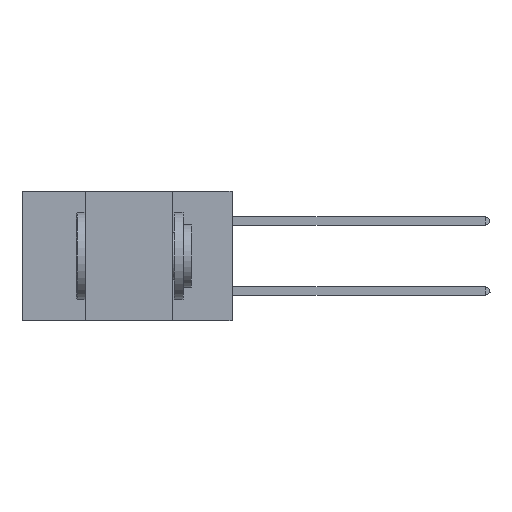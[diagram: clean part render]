
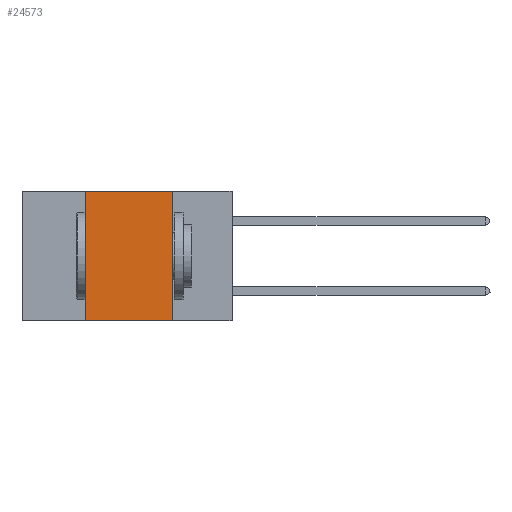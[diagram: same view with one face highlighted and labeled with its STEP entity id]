
A CAD part, left-side view. The second image highlights one B-rep face of the part: STEP entity #24573.
In plain terms, the highlighted planar face has unit normal (-1, 0, 0).
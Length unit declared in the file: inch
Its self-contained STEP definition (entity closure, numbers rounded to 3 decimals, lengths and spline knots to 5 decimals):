
#887 = CARTESIAN_POINT ( 'NONE',  ( 0., 0.42, -0.37 ) ) ;
#1390 = FACE_OUTER_BOUND ( 'NONE', #9276, .T. ) ;
#1487 = ORIENTED_EDGE ( 'NONE', *, *, #33273, .F. ) ;
#3387 = CARTESIAN_POINT ( 'NONE',  ( 0., 0.6, -0.37 ) ) ;
#4075 = VERTEX_POINT ( 'NONE', #34671 ) ;
#4514 = DIRECTION ( 'NONE',  ( 0., -1., 0. ) ) ;
#5145 = LINE ( 'NONE', #28663, #33664 ) ;
#7733 = DIRECTION ( 'NONE',  ( 0., 0., -1. ) ) ;
#7948 = VERTEX_POINT ( 'NONE', #12172 ) ;
#8188 = LINE ( 'NONE', #35156, #29239 ) ;
#9276 = EDGE_LOOP ( 'NONE', ( #1487, #20890, #13299, #32696 ) ) ;
#9795 = DIRECTION ( 'NONE',  ( 0., 0., 1. ) ) ;
#12172 = CARTESIAN_POINT ( 'NONE',  ( 0., 0.17, -0.37 ) ) ;
#13299 = ORIENTED_EDGE ( 'NONE', *, *, #27723, .F. ) ;
#16791 = DIRECTION ( 'NONE',  ( 0., 0., -1. ) ) ;
#17691 = VERTEX_POINT ( 'NONE', #887 ) ;
#17875 = LINE ( 'NONE', #3387, #32111 ) ;
#17896 = CARTESIAN_POINT ( 'NONE',  ( 0., 0.6, 0. ) ) ;
#18931 = EDGE_CURVE ( 'NONE', #4075, #21295, #27605, .T. ) ;
#20890 = ORIENTED_EDGE ( 'NONE', *, *, #18931, .F. ) ;
#21270 = AXIS2_PLACEMENT_3D ( 'NONE', #24106, #21484, #7733 ) ;
#21295 = VERTEX_POINT ( 'NONE', #23881 ) ;
#21484 = DIRECTION ( 'NONE',  ( 1., 0., 0. ) ) ;
#22049 = VECTOR ( 'NONE', #4514, 39.37008 ) ;
#22557 = EDGE_CURVE ( 'NONE', #17691, #7948, #17875, .T. ) ;
#23881 = CARTESIAN_POINT ( 'NONE',  ( 0., 0.17, 0. ) ) ;
#24106 = CARTESIAN_POINT ( 'NONE',  ( 0., 0.6, 0. ) ) ;
#24573 = ADVANCED_FACE ( 'NONE', ( #1390 ), #32306, .F. ) ;
#25418 = DIRECTION ( 'NONE',  ( 0., -1., 0. ) ) ;
#27605 = LINE ( 'NONE', #17896, #22049 ) ;
#27723 = EDGE_CURVE ( 'NONE', #17691, #4075, #5145, .T. ) ;
#28663 = CARTESIAN_POINT ( 'NONE',  ( 0., 0.42, 0. ) ) ;
#29239 = VECTOR ( 'NONE', #16791, 39.37008 ) ;
#32111 = VECTOR ( 'NONE', #25418, 39.37008 ) ;
#32306 = PLANE ( 'NONE',  #21270 ) ;
#32696 = ORIENTED_EDGE ( 'NONE', *, *, #22557, .T. ) ;
#33273 = EDGE_CURVE ( 'NONE', #21295, #7948, #8188, .T. ) ;
#33664 = VECTOR ( 'NONE', #9795, 39.37008 ) ;
#34671 = CARTESIAN_POINT ( 'NONE',  ( 0., 0.42, 0. ) ) ;
#35156 = CARTESIAN_POINT ( 'NONE',  ( 0., 0.17, 0. ) ) ;
